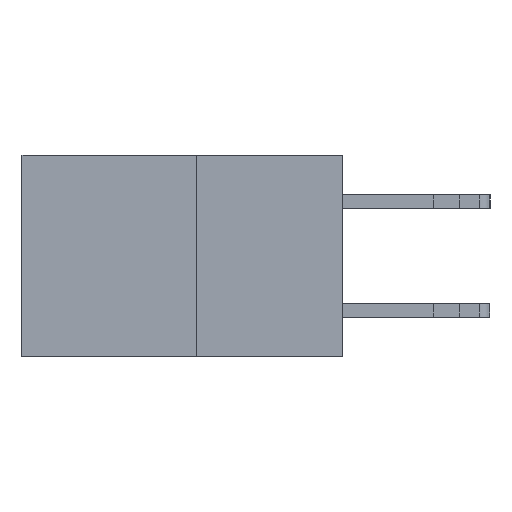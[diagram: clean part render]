
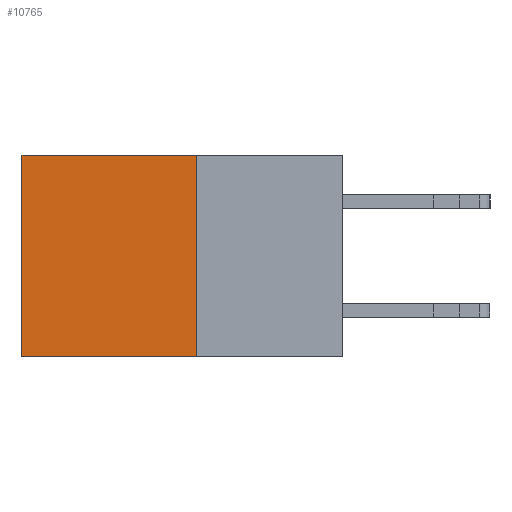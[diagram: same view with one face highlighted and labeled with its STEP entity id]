
A CAD part, left-side view. The second image highlights one B-rep face of the part: STEP entity #10765.
In plain terms, the highlighted planar face has unit normal (-1, 0, 0).
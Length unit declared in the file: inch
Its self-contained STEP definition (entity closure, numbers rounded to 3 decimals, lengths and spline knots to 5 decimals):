
#70 = AXIS2_PLACEMENT_3D ( 'NONE', #6706, #624, #9171 ) ;
#83 = CARTESIAN_POINT ( 'NONE',  ( 0.277, 0.27, -0.37 ) ) ;
#229 = FACE_OUTER_BOUND ( 'NONE', #14742, .T. ) ;
#624 = DIRECTION ( 'NONE',  ( 1., 0., 0. ) ) ;
#662 = LINE ( 'NONE', #83, #10024 ) ;
#1453 = ORIENTED_EDGE ( 'NONE', *, *, #3387, .F. ) ;
#1506 = CARTESIAN_POINT ( 'NONE',  ( 0.277, 0.59, -0.37 ) ) ;
#1841 = ORIENTED_EDGE ( 'NONE', *, *, #15306, .T. ) ;
#2551 = VECTOR ( 'NONE', #12538, 39.37008 ) ;
#2791 = VECTOR ( 'NONE', #12793, 39.37008 ) ;
#3387 = EDGE_CURVE ( 'NONE', #6951, #6351, #3579, .T. ) ;
#3579 = LINE ( 'NONE', #7733, #2791 ) ;
#3908 = CARTESIAN_POINT ( 'NONE',  ( 0.277, 0.27, 0. ) ) ;
#4552 = LINE ( 'NONE', #12933, #13350 ) ;
#4824 = ORIENTED_EDGE ( 'NONE', *, *, #5177, .T. ) ;
#5177 = EDGE_CURVE ( 'NONE', #12443, #12095, #5767, .T. ) ;
#5767 = LINE ( 'NONE', #15606, #2551 ) ;
#6351 = VERTEX_POINT ( 'NONE', #1506 ) ;
#6598 = ORIENTED_EDGE ( 'NONE', *, *, #8307, .F. ) ;
#6706 = CARTESIAN_POINT ( 'NONE',  ( 0.277, 0.27, -0.37 ) ) ;
#6951 = VERTEX_POINT ( 'NONE', #9844 ) ;
#7733 = CARTESIAN_POINT ( 'NONE',  ( 0.277, 0.27, -0.37 ) ) ;
#8307 = EDGE_CURVE ( 'NONE', #12443, #6951, #662, .T. ) ;
#9171 = DIRECTION ( 'NONE',  ( 0., 0., -1. ) ) ;
#9844 = CARTESIAN_POINT ( 'NONE',  ( 0.277, 0.27, -0.37 ) ) ;
#10024 = VECTOR ( 'NONE', #13363, 39.37008 ) ;
#10765 = ADVANCED_FACE ( 'NONE', ( #229 ), #15111, .F. ) ;
#12095 = VERTEX_POINT ( 'NONE', #14018 ) ;
#12443 = VERTEX_POINT ( 'NONE', #3908 ) ;
#12538 = DIRECTION ( 'NONE',  ( 0., 1., 0. ) ) ;
#12793 = DIRECTION ( 'NONE',  ( 0., 1., 0. ) ) ;
#12933 = CARTESIAN_POINT ( 'NONE',  ( 0.277, 0.59, -0.37 ) ) ;
#13350 = VECTOR ( 'NONE', #14139, 39.37008 ) ;
#13363 = DIRECTION ( 'NONE',  ( 0., 0., -1. ) ) ;
#14018 = CARTESIAN_POINT ( 'NONE',  ( 0.277, 0.59, 0. ) ) ;
#14139 = DIRECTION ( 'NONE',  ( 0., 0., -1. ) ) ;
#14742 = EDGE_LOOP ( 'NONE', ( #1841, #1453, #6598, #4824 ) ) ;
#15111 = PLANE ( 'NONE',  #70 ) ;
#15306 = EDGE_CURVE ( 'NONE', #12095, #6351, #4552, .T. ) ;
#15606 = CARTESIAN_POINT ( 'NONE',  ( 0.277, 0.27, 0. ) ) ;
